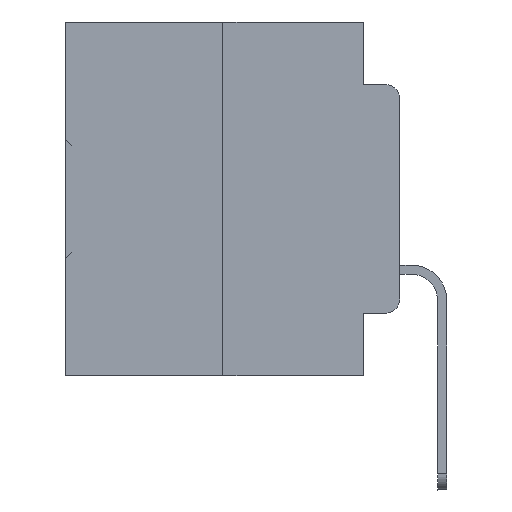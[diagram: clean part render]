
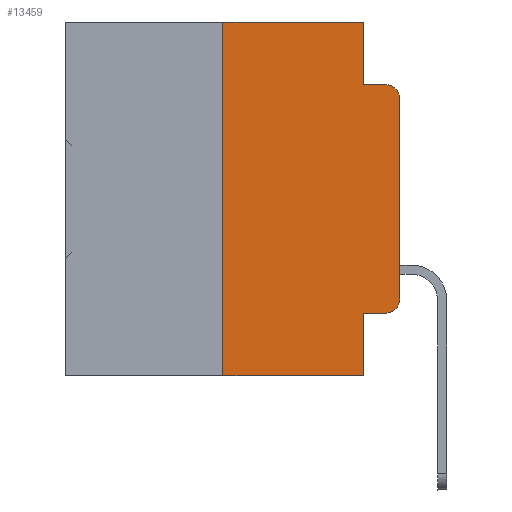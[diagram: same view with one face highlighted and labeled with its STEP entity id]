
A CAD part, left-side view. The second image highlights one B-rep face of the part: STEP entity #13459.
In plain terms, the highlighted planar face has unit normal (-1, 0, 0).
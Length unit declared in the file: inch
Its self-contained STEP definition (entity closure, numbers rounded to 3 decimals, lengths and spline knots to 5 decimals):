
#634 = ORIENTED_EDGE ( 'NONE', *, *, #17612, .F. ) ;
#1349 = CARTESIAN_POINT ( 'NONE',  ( 0., 0.02, -0.4115 ) ) ;
#1382 = ORIENTED_EDGE ( 'NONE', *, *, #34053, .T. ) ;
#1520 = CARTESIAN_POINT ( 'NONE',  ( 0., 0.02, -0.0885 ) ) ;
#1532 = DIRECTION ( 'NONE',  ( 1., 0., 0. ) ) ;
#1770 = LINE ( 'NONE', #24953, #30316 ) ;
#2033 = ORIENTED_EDGE ( 'NONE', *, *, #11731, .T. ) ;
#2632 = CARTESIAN_POINT ( 'NONE',  ( 0., 0.473, -0.5 ) ) ;
#2712 = VERTEX_POINT ( 'NONE', #9135 ) ;
#2772 = CARTESIAN_POINT ( 'NONE',  ( 0., 0.473, 0. ) ) ;
#2816 = CARTESIAN_POINT ( 'NONE',  ( 0., 0.25, -0.5 ) ) ;
#2852 = CARTESIAN_POINT ( 'NONE',  ( 0., 0.02, -0.1085 ) ) ;
#3343 = EDGE_CURVE ( 'NONE', #2712, #32108, #24723, .T. ) ;
#3876 = DIRECTION ( 'NONE',  ( 0., 0., 1. ) ) ;
#4128 = VECTOR ( 'NONE', #21414, 39.37008 ) ;
#4193 = LINE ( 'NONE', #23663, #21078 ) ;
#4705 = AXIS2_PLACEMENT_3D ( 'NONE', #19831, #31359, #23042 ) ;
#5110 = ORIENTED_EDGE ( 'NONE', *, *, #9149, .T. ) ;
#5703 = DIRECTION ( 'NONE',  ( 0., -1., 0. ) ) ;
#6935 = VECTOR ( 'NONE', #33941, 39.37008 ) ;
#7802 = ORIENTED_EDGE ( 'NONE', *, *, #28897, .F. ) ;
#8110 = LINE ( 'NONE', #2632, #6935 ) ;
#8261 = VECTOR ( 'NONE', #13895, 39.37008 ) ;
#8479 = AXIS2_PLACEMENT_3D ( 'NONE', #2852, #23204, #34731 ) ;
#9135 = CARTESIAN_POINT ( 'NONE',  ( 0., 0., -0.1085 ) ) ;
#9149 = EDGE_CURVE ( 'NONE', #36475, #23602, #25778, .T. ) ;
#9207 = ORIENTED_EDGE ( 'NONE', *, *, #30848, .F. ) ;
#9933 = LINE ( 'NONE', #13131, #4128 ) ;
#11169 = CARTESIAN_POINT ( 'NONE',  ( 0., 0.051, -0.0885 ) ) ;
#11460 = LINE ( 'NONE', #34467, #36560 ) ;
#11465 = CARTESIAN_POINT ( 'NONE',  ( 0., 0.051, -0.5 ) ) ;
#11731 = EDGE_CURVE ( 'NONE', #28509, #36927, #8110, .T. ) ;
#13009 = CARTESIAN_POINT ( 'NONE',  ( 0., 0.051, -0.0885 ) ) ;
#13027 = DIRECTION ( 'NONE',  ( 0., 0., -1. ) ) ;
#13131 = CARTESIAN_POINT ( 'NONE',  ( 0., 0.051, -0.4115 ) ) ;
#13459 = ADVANCED_FACE ( 'NONE', ( #27346 ), #33219, .F. ) ;
#13895 = DIRECTION ( 'NONE',  ( 0., -1., 0. ) ) ;
#14118 = EDGE_LOOP ( 'NONE', ( #1382, #26843, #27149, #9207, #7802, #31433, #2033, #634, #20965, #5110 ) ) ;
#16118 = CARTESIAN_POINT ( 'NONE',  ( 0., 0., -0.3915 ) ) ;
#17059 = LINE ( 'NONE', #2772, #8261 ) ;
#17265 = DIRECTION ( 'NONE',  ( 0., 0., 1. ) ) ;
#17612 = EDGE_CURVE ( 'NONE', #36858, #36927, #4193, .T. ) ;
#19831 = CARTESIAN_POINT ( 'NONE',  ( 0., 0.02, -0.3915 ) ) ;
#20005 = LINE ( 'NONE', #11169, #34780 ) ;
#20412 = CARTESIAN_POINT ( 'NONE',  ( 0., 0.051, 0. ) ) ;
#20849 = VERTEX_POINT ( 'NONE', #28960 ) ;
#20965 = ORIENTED_EDGE ( 'NONE', *, *, #37297, .T. ) ;
#21078 = VECTOR ( 'NONE', #27371, 39.37008 ) ;
#21414 = DIRECTION ( 'NONE',  ( 0., -1., 0. ) ) ;
#22003 = VERTEX_POINT ( 'NONE', #13009 ) ;
#23042 = DIRECTION ( 'NONE',  ( 0., 0., -1. ) ) ;
#23204 = DIRECTION ( 'NONE',  ( -1., 0., 0. ) ) ;
#23602 = VERTEX_POINT ( 'NONE', #16118 ) ;
#23663 = CARTESIAN_POINT ( 'NONE',  ( 0., 0.051, 0. ) ) ;
#24723 = CIRCLE ( 'NONE', #8479, 0.02 ) ;
#24953 = CARTESIAN_POINT ( 'NONE',  ( 0., 0.051, 0. ) ) ;
#25778 = CIRCLE ( 'NONE', #4705, 0.02 ) ;
#26843 = ORIENTED_EDGE ( 'NONE', *, *, #3343, .T. ) ;
#26849 = VECTOR ( 'NONE', #3876, 39.37008 ) ;
#26945 = VERTEX_POINT ( 'NONE', #20412 ) ;
#27149 = ORIENTED_EDGE ( 'NONE', *, *, #34583, .F. ) ;
#27346 = FACE_OUTER_BOUND ( 'NONE', #14118, .T. ) ;
#27371 = DIRECTION ( 'NONE',  ( 0., 0., -1. ) ) ;
#27497 = CARTESIAN_POINT ( 'NONE',  ( 0., 0.051, -0.4115 ) ) ;
#27772 = EDGE_CURVE ( 'NONE', #28509, #20849, #29710, .T. ) ;
#28509 = VERTEX_POINT ( 'NONE', #2816 ) ;
#28897 = EDGE_CURVE ( 'NONE', #20849, #26945, #17059, .T. ) ;
#28960 = CARTESIAN_POINT ( 'NONE',  ( 0., 0.25, 0. ) ) ;
#29710 = LINE ( 'NONE', #35193, #26849 ) ;
#30316 = VECTOR ( 'NONE', #36284, 39.37008 ) ;
#30546 = AXIS2_PLACEMENT_3D ( 'NONE', #33030, #1532, #13027 ) ;
#30848 = EDGE_CURVE ( 'NONE', #26945, #22003, #1770, .T. ) ;
#31359 = DIRECTION ( 'NONE',  ( -1., 0., 0. ) ) ;
#31433 = ORIENTED_EDGE ( 'NONE', *, *, #27772, .F. ) ;
#32108 = VERTEX_POINT ( 'NONE', #1520 ) ;
#33030 = CARTESIAN_POINT ( 'NONE',  ( 0., 0.473, 0. ) ) ;
#33219 = PLANE ( 'NONE',  #30546 ) ;
#33941 = DIRECTION ( 'NONE',  ( 0., -1., 0. ) ) ;
#34053 = EDGE_CURVE ( 'NONE', #23602, #2712, #11460, .T. ) ;
#34467 = CARTESIAN_POINT ( 'NONE',  ( 0., 0., 0. ) ) ;
#34583 = EDGE_CURVE ( 'NONE', #22003, #32108, #20005, .T. ) ;
#34731 = DIRECTION ( 'NONE',  ( 0., 0., -1. ) ) ;
#34780 = VECTOR ( 'NONE', #5703, 39.37008 ) ;
#35193 = CARTESIAN_POINT ( 'NONE',  ( 0., 0.25, 0. ) ) ;
#36284 = DIRECTION ( 'NONE',  ( 0., 0., -1. ) ) ;
#36475 = VERTEX_POINT ( 'NONE', #1349 ) ;
#36560 = VECTOR ( 'NONE', #17265, 39.37008 ) ;
#36858 = VERTEX_POINT ( 'NONE', #27497 ) ;
#36927 = VERTEX_POINT ( 'NONE', #11465 ) ;
#37297 = EDGE_CURVE ( 'NONE', #36858, #36475, #9933, .T. ) ;
